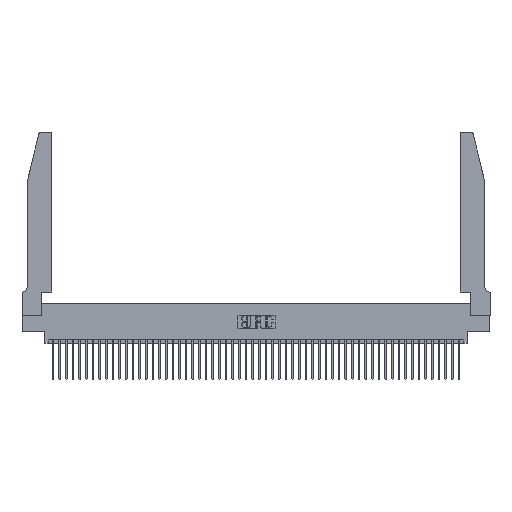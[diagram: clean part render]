
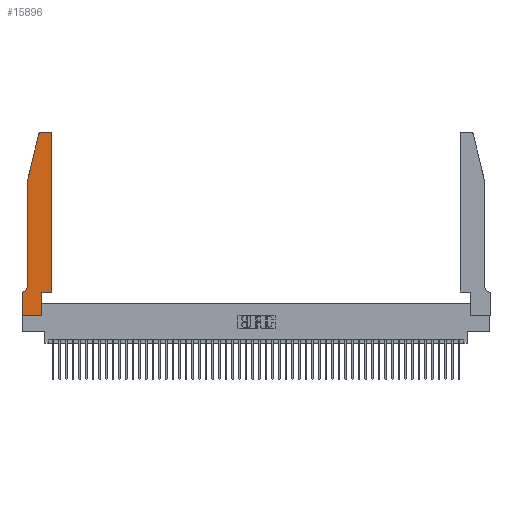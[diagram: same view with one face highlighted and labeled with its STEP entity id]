
A CAD part, top view. The second image highlights one B-rep face of the part: STEP entity #15896.
In plain terms, the highlighted planar face has unit normal (0, 0, 1).
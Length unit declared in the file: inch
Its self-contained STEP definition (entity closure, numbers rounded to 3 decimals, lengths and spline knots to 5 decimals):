
#18 = LINE ( 'NONE', #49867, #49832 ) ;
#233 = ORIENTED_EDGE ( 'NONE', *, *, #41094, .T. ) ;
#738 = DIRECTION ( 'NONE',  ( 0., 1., 0. ) ) ;
#1220 = ORIENTED_EDGE ( 'NONE', *, *, #2099, .T. ) ;
#1293 = CIRCLE ( 'NONE', #48583, 0.07 ) ;
#1769 = VERTEX_POINT ( 'NONE', #27361 ) ;
#2088 = CARTESIAN_POINT ( 'NONE',  ( 0., 0.35, 0.37 ) ) ;
#2099 = EDGE_CURVE ( 'NONE', #1769, #32781, #3973, .T. ) ;
#2172 = EDGE_CURVE ( 'NONE', #32781, #40466, #10917, .T. ) ;
#2378 = DIRECTION ( 'NONE',  ( 0., -1., 0. ) ) ;
#3018 = DIRECTION ( 'NONE',  ( -1., 0., 0. ) ) ;
#3050 = VECTOR ( 'NONE', #738, 39.37008 ) ;
#3973 = LINE ( 'NONE', #17577, #6514 ) ;
#4275 = VERTEX_POINT ( 'NONE', #19765 ) ;
#4735 = DIRECTION ( 'NONE',  ( -1., 0., 0. ) ) ;
#4845 = EDGE_CURVE ( 'NONE', #4275, #1769, #18, .T. ) ;
#6165 = EDGE_CURVE ( 'NONE', #28713, #48100, #22300, .T. ) ;
#6297 = DIRECTION ( 'NONE',  ( 1., 0., 0. ) ) ;
#6514 = VECTOR ( 'NONE', #48741, 39.37008 ) ;
#9286 = DIRECTION ( 'NONE',  ( -0.239, -0.971, 0. ) ) ;
#10476 = DIRECTION ( 'NONE',  ( 0., 0., 1. ) ) ;
#10810 = CARTESIAN_POINT ( 'NONE',  ( 0.4505, 0.35, 0.37 ) ) ;
#10917 = LINE ( 'NONE', #10810, #12155 ) ;
#10938 = VERTEX_POINT ( 'NONE', #35819 ) ;
#11050 = ORIENTED_EDGE ( 'NONE', *, *, #4845, .T. ) ;
#12155 = VECTOR ( 'NONE', #42124, 39.37008 ) ;
#12558 = VECTOR ( 'NONE', #2378, 39.37008 ) ;
#12608 = ORIENTED_EDGE ( 'NONE', *, *, #34336, .T. ) ;
#13061 = VECTOR ( 'NONE', #9286, 39.37008 ) ;
#13803 = ORIENTED_EDGE ( 'NONE', *, *, #33336, .T. ) ;
#13990 = CARTESIAN_POINT ( 'NONE',  ( 0.4505, 2.72, 0.37 ) ) ;
#14682 = AXIS2_PLACEMENT_3D ( 'NONE', #33972, #10476, #37905 ) ;
#15299 = ORIENTED_EDGE ( 'NONE', *, *, #2172, .T. ) ;
#15302 = VERTEX_POINT ( 'NONE', #26768 ) ;
#15896 = ADVANCED_FACE ( 'NONE', ( #22043 ), #22125, .T. ) ;
#16109 = CARTESIAN_POINT ( 'NONE',  ( 0.0755, 2., 0.37 ) ) ;
#16338 = AXIS2_PLACEMENT_3D ( 'NONE', #20581, #47784, #24501 ) ;
#17420 = CIRCLE ( 'NONE', #14682, 0.03 ) ;
#17577 = CARTESIAN_POINT ( 'NONE',  ( 0.2865, 0.35, 0.37 ) ) ;
#17592 = CARTESIAN_POINT ( 'NONE',  ( 0.4205, 2.75, 0.37 ) ) ;
#17717 = DIRECTION ( 'NONE',  ( 0., -1., 0. ) ) ;
#18414 = ORIENTED_EDGE ( 'NONE', *, *, #19692, .T. ) ;
#19297 = EDGE_CURVE ( 'NONE', #40466, #26755, #34545, .T. ) ;
#19692 = EDGE_CURVE ( 'NONE', #26755, #31301, #17420, .T. ) ;
#19765 = CARTESIAN_POINT ( 'NONE',  ( 0., 0., 0.37 ) ) ;
#20581 = CARTESIAN_POINT ( 'NONE',  ( 0.284, 2.72, 0.37 ) ) ;
#20792 = CARTESIAN_POINT ( 'NONE',  ( 0.0755, 0.35, 0.37 ) ) ;
#21344 = VECTOR ( 'NONE', #48637, 39.37008 ) ;
#22043 = FACE_OUTER_BOUND ( 'NONE', #44255, .T. ) ;
#22125 = PLANE ( 'NONE',  #30386 ) ;
#22300 = LINE ( 'NONE', #36747, #13061 ) ;
#22572 = LINE ( 'NONE', #44720, #21344 ) ;
#22660 = DIRECTION ( 'NONE',  ( 1., 0., 0. ) ) ;
#23285 = CARTESIAN_POINT ( 'NONE',  ( 0.4505, 0.35, 0.37 ) ) ;
#23451 = LINE ( 'NONE', #37145, #32549 ) ;
#24501 = DIRECTION ( 'NONE',  ( 1., 0., 0. ) ) ;
#25462 = LINE ( 'NONE', #20792, #47350 ) ;
#25979 = ORIENTED_EDGE ( 'NONE', *, *, #30077, .T. ) ;
#26755 = VERTEX_POINT ( 'NONE', #13990 ) ;
#26768 = CARTESIAN_POINT ( 'NONE',  ( 0.284, 2.75, 0.37 ) ) ;
#26789 = DIRECTION ( 'NONE',  ( 0., 0., -1. ) ) ;
#26902 = ORIENTED_EDGE ( 'NONE', *, *, #6165, .T. ) ;
#27361 = CARTESIAN_POINT ( 'NONE',  ( 0.2865, 0., 0.37 ) ) ;
#28713 = VERTEX_POINT ( 'NONE', #38442 ) ;
#29942 = DIRECTION ( 'NONE',  ( 0., 0., 1. ) ) ;
#30077 = EDGE_CURVE ( 'NONE', #48100, #47087, #23451, .T. ) ;
#30386 = AXIS2_PLACEMENT_3D ( 'NONE', #2088, #29942, #6297 ) ;
#31301 = VERTEX_POINT ( 'NONE', #17592 ) ;
#31698 = CARTESIAN_POINT ( 'NONE',  ( 0.0755, 0.42, 0.37 ) ) ;
#32549 = VECTOR ( 'NONE', #17717, 39.37008 ) ;
#32781 = VERTEX_POINT ( 'NONE', #42039 ) ;
#33336 = EDGE_CURVE ( 'NONE', #47771, #4275, #42536, .T. ) ;
#33972 = CARTESIAN_POINT ( 'NONE',  ( 0.4205, 2.72, 0.37 ) ) ;
#34336 = EDGE_CURVE ( 'NONE', #10938, #47771, #25462, .T. ) ;
#34545 = LINE ( 'NONE', #47106, #3050 ) ;
#35819 = CARTESIAN_POINT ( 'NONE',  ( 0.0055, 0.35, 0.37 ) ) ;
#36014 = ORIENTED_EDGE ( 'NONE', *, *, #19297, .T. ) ;
#36747 = CARTESIAN_POINT ( 'NONE',  ( 0.0755, 2., 0.37 ) ) ;
#37145 = CARTESIAN_POINT ( 'NONE',  ( 0.0755, 2., 0.37 ) ) ;
#37489 = CIRCLE ( 'NONE', #16338, 0.03 ) ;
#37905 = DIRECTION ( 'NONE',  ( 1., 0., 0. ) ) ;
#38442 = CARTESIAN_POINT ( 'NONE',  ( 0.25487, 2.72718, 0.37 ) ) ;
#40122 = EDGE_CURVE ( 'NONE', #31301, #15302, #22572, .T. ) ;
#40466 = VERTEX_POINT ( 'NONE', #23285 ) ;
#41094 = EDGE_CURVE ( 'NONE', #47087, #10938, #1293, .T. ) ;
#41573 = CARTESIAN_POINT ( 'NONE',  ( 0., 0.35, 0.37 ) ) ;
#42039 = CARTESIAN_POINT ( 'NONE',  ( 0.2865, 0.35, 0.37 ) ) ;
#42124 = DIRECTION ( 'NONE',  ( 1., 0., 0. ) ) ;
#42536 = LINE ( 'NONE', #49465, #12558 ) ;
#43109 = ORIENTED_EDGE ( 'NONE', *, *, #40122, .T. ) ;
#43546 = ORIENTED_EDGE ( 'NONE', *, *, #43902, .T. ) ;
#43902 = EDGE_CURVE ( 'NONE', #15302, #28713, #37489, .T. ) ;
#44255 = EDGE_LOOP ( 'NONE', ( #43109, #43546, #26902, #25979, #233, #12608, #13803, #11050, #1220, #15299, #36014, #18414 ) ) ;
#44720 = CARTESIAN_POINT ( 'NONE',  ( 0.2605, 2.75, 0.37 ) ) ;
#47087 = VERTEX_POINT ( 'NONE', #31698 ) ;
#47106 = CARTESIAN_POINT ( 'NONE',  ( 0.4505, 0.35, 0.37 ) ) ;
#47350 = VECTOR ( 'NONE', #4735, 39.37008 ) ;
#47771 = VERTEX_POINT ( 'NONE', #41573 ) ;
#47784 = DIRECTION ( 'NONE',  ( 0., 0., 1. ) ) ;
#48100 = VERTEX_POINT ( 'NONE', #16109 ) ;
#48583 = AXIS2_PLACEMENT_3D ( 'NONE', #50091, #26789, #3018 ) ;
#48637 = DIRECTION ( 'NONE',  ( -1., 0., 0. ) ) ;
#48741 = DIRECTION ( 'NONE',  ( 0., 1., 0. ) ) ;
#49465 = CARTESIAN_POINT ( 'NONE',  ( 0., 0., 0.37 ) ) ;
#49832 = VECTOR ( 'NONE', #22660, 39.37008 ) ;
#49867 = CARTESIAN_POINT ( 'NONE',  ( 0., 0., 0.37 ) ) ;
#50091 = CARTESIAN_POINT ( 'NONE',  ( 0.0055, 0.42, 0.37 ) ) ;
